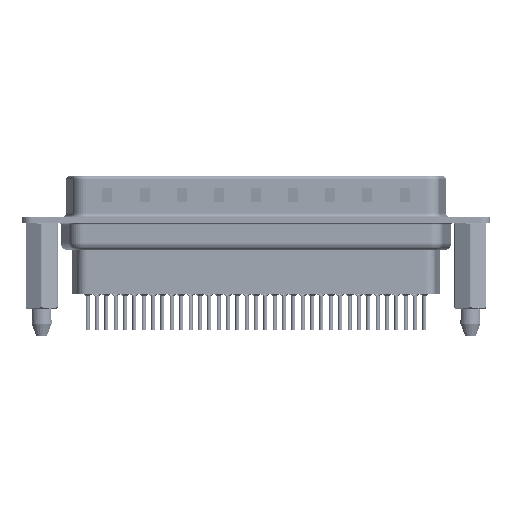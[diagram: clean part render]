
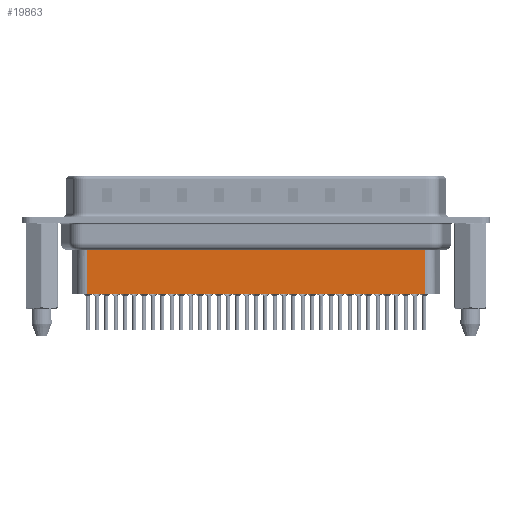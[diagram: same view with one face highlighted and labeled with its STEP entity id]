
A CAD part, front view. The second image highlights one B-rep face of the part: STEP entity #19863.
In plain terms, the highlighted planar face has unit normal (0, -1, 0).
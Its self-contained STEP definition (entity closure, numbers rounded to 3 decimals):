
#118 = FACE_OUTER_BOUND ( 'NONE', #21409, .T. ) ;
#568 = VERTEX_POINT ( 'NONE', #28003 ) ;
#633 = ORIENTED_EDGE ( 'NONE', *, *, #16168, .T. ) ;
#710 = EDGE_CURVE ( 'NONE', #21749, #18518, #9364, .T. ) ;
#2230 = CARTESIAN_POINT ( 'NONE',  ( 56.794, -3.5, -3.1 ) ) ;
#2401 = CARTESIAN_POINT ( 'NONE',  ( 6.706, -3.5, -10.95 ) ) ;
#4131 = CARTESIAN_POINT ( 'NONE',  ( 56.794, -3.5, -10.95 ) ) ;
#4750 = VECTOR ( 'NONE', #30168, 1000. ) ;
#5502 = DIRECTION ( 'NONE',  ( 0., -1., 0. ) ) ;
#6940 = DIRECTION ( 'NONE',  ( 0., 0., -1. ) ) ;
#7030 = ORIENTED_EDGE ( 'NONE', *, *, #710, .F. ) ;
#7723 = ORIENTED_EDGE ( 'NONE', *, *, #25889, .F. ) ;
#8193 = VECTOR ( 'NONE', #19411, 1000. ) ;
#8825 = CARTESIAN_POINT ( 'NONE',  ( 56.794, -3.5, -4.097 ) ) ;
#9364 = LINE ( 'NONE', #2230, #13917 ) ;
#11034 = EDGE_CURVE ( 'NONE', #21749, #568, #22185, .T. ) ;
#12650 = AXIS2_PLACEMENT_3D ( 'NONE', #29745, #5502, #15390 ) ;
#13545 = VERTEX_POINT ( 'NONE', #24833 ) ;
#13917 = VECTOR ( 'NONE', #6940, 1000. ) ;
#15003 = LINE ( 'NONE', #28043, #4750 ) ;
#15390 = DIRECTION ( 'NONE',  ( 1., 0., 0. ) ) ;
#16168 = EDGE_CURVE ( 'NONE', #568, #13545, #15003, .T. ) ;
#18014 = VECTOR ( 'NONE', #29575, 1000. ) ;
#18518 = VERTEX_POINT ( 'NONE', #4131 ) ;
#19411 = DIRECTION ( 'NONE',  ( -1., 0., 0. ) ) ;
#19606 = LINE ( 'NONE', #2401, #18014 ) ;
#19773 = PLANE ( 'NONE',  #12650 ) ;
#19863 = ADVANCED_FACE ( 'NONE', ( #118 ), #19773, .T. ) ;
#21409 = EDGE_LOOP ( 'NONE', ( #7030, #26133, #633, #7723 ) ) ;
#21713 = CARTESIAN_POINT ( 'NONE',  ( 6.459, -3.5, -4.097 ) ) ;
#21749 = VERTEX_POINT ( 'NONE', #8825 ) ;
#22185 = LINE ( 'NONE', #21713, #8193 ) ;
#24833 = CARTESIAN_POINT ( 'NONE',  ( 6.706, -3.5, -10.95 ) ) ;
#25889 = EDGE_CURVE ( 'NONE', #18518, #13545, #19606, .T. ) ;
#26133 = ORIENTED_EDGE ( 'NONE', *, *, #11034, .T. ) ;
#28003 = CARTESIAN_POINT ( 'NONE',  ( 6.706, -3.5, -4.097 ) ) ;
#28043 = CARTESIAN_POINT ( 'NONE',  ( 6.706, -3.5, -3.1 ) ) ;
#29575 = DIRECTION ( 'NONE',  ( -1., 0., 0. ) ) ;
#29745 = CARTESIAN_POINT ( 'NONE',  ( 6.706, -3.5, -3.1 ) ) ;
#30168 = DIRECTION ( 'NONE',  ( 0., 0., -1. ) ) ;
